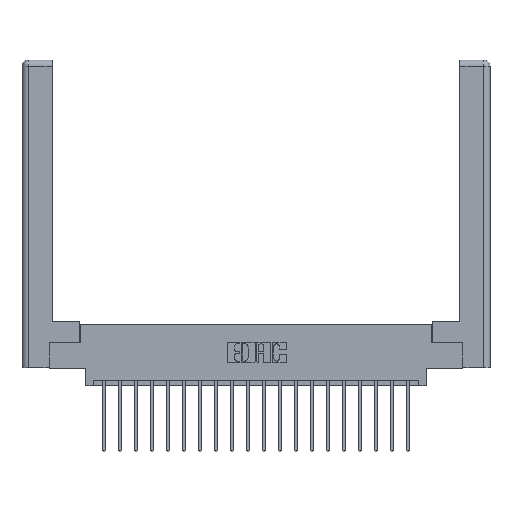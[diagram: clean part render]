
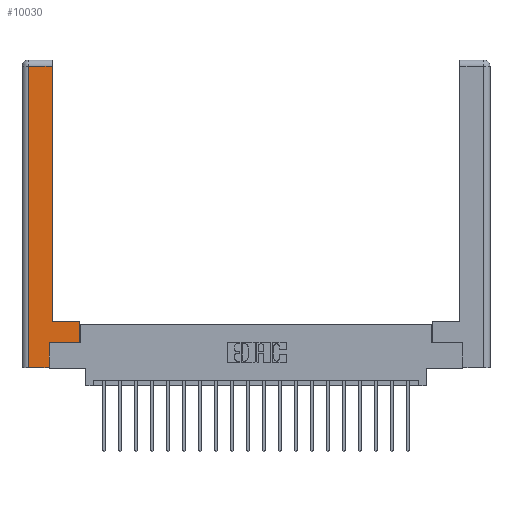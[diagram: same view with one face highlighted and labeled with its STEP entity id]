
A CAD part, top view. The second image highlights one B-rep face of the part: STEP entity #10030.
In plain terms, the highlighted planar face has unit normal (0, 0, 1).
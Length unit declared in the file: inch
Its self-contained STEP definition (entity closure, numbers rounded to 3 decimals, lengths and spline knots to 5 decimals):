
#291 = CARTESIAN_POINT ( 'NONE',  ( 0.265, 0.245, 0. ) ) ;
#354 = VECTOR ( 'NONE', #7674, 39.37008 ) ;
#546 = CARTESIAN_POINT ( 'NONE',  ( 0.0615, 2.94, 0. ) ) ;
#1181 = PLANE ( 'NONE',  #9428 ) ;
#1514 = EDGE_CURVE ( 'NONE', #5510, #20855, #13530, .T. ) ;
#1577 = CARTESIAN_POINT ( 'NONE',  ( 0.295, 2.94, 0. ) ) ;
#1755 = VERTEX_POINT ( 'NONE', #2983 ) ;
#2409 = CARTESIAN_POINT ( 'NONE',  ( 0.265, 0., 0. ) ) ;
#2496 = ORIENTED_EDGE ( 'NONE', *, *, #8917, .T. ) ;
#2958 = VERTEX_POINT ( 'NONE', #291 ) ;
#2983 = CARTESIAN_POINT ( 'NONE',  ( 0.295, 0.45, 0. ) ) ;
#3250 = LINE ( 'NONE', #9101, #7312 ) ;
#3338 = VECTOR ( 'NONE', #19075, 39.37008 ) ;
#3557 = CARTESIAN_POINT ( 'NONE',  ( 0.265, 0., 0. ) ) ;
#3726 = ORIENTED_EDGE ( 'NONE', *, *, #14998, .T. ) ;
#3852 = LINE ( 'NONE', #12488, #3338 ) ;
#4412 = DIRECTION ( 'NONE',  ( 0., 1., 0. ) ) ;
#4414 = DIRECTION ( 'NONE',  ( -1., 0., 0. ) ) ;
#4486 = DIRECTION ( 'NONE',  ( 0., 0., -1. ) ) ;
#4627 = LINE ( 'NONE', #19102, #10732 ) ;
#5510 = VERTEX_POINT ( 'NONE', #15544 ) ;
#5844 = VERTEX_POINT ( 'NONE', #11679 ) ;
#6063 = FACE_OUTER_BOUND ( 'NONE', #18761, .T. ) ;
#6255 = ORIENTED_EDGE ( 'NONE', *, *, #10693, .T. ) ;
#6466 = DIRECTION ( 'NONE',  ( 0., -1., 0. ) ) ;
#6658 = ORIENTED_EDGE ( 'NONE', *, *, #1514, .T. ) ;
#7312 = VECTOR ( 'NONE', #4412, 39.37008 ) ;
#7674 = DIRECTION ( 'NONE',  ( 0., 1., 0. ) ) ;
#8018 = LINE ( 'NONE', #9523, #354 ) ;
#8917 = EDGE_CURVE ( 'NONE', #2958, #19287, #4627, .T. ) ;
#9101 = CARTESIAN_POINT ( 'NONE',  ( 0.565, 0.45, 0. ) ) ;
#9197 = VECTOR ( 'NONE', #13672, 39.37008 ) ;
#9251 = VECTOR ( 'NONE', #16323, 39.37008 ) ;
#9428 = AXIS2_PLACEMENT_3D ( 'NONE', #10957, #4486, #4414 ) ;
#9523 = CARTESIAN_POINT ( 'NONE',  ( 0.295, 3., 0. ) ) ;
#9700 = VECTOR ( 'NONE', #14071, 39.37008 ) ;
#10030 = ADVANCED_FACE ( 'NONE', ( #6063 ), #1181, .F. ) ;
#10693 = EDGE_CURVE ( 'NONE', #19287, #5844, #3250, .T. ) ;
#10732 = VECTOR ( 'NONE', #12814, 39.37008 ) ;
#10761 = ORIENTED_EDGE ( 'NONE', *, *, #15129, .T. ) ;
#10957 = CARTESIAN_POINT ( 'NONE',  ( 0., 0., 0. ) ) ;
#11517 = CARTESIAN_POINT ( 'NONE',  ( 0.565, 0.245, 0. ) ) ;
#11679 = CARTESIAN_POINT ( 'NONE',  ( 0.565, 0.45, 0. ) ) ;
#12003 = EDGE_CURVE ( 'NONE', #1755, #14432, #8018, .T. ) ;
#12488 = CARTESIAN_POINT ( 'NONE',  ( 0.265, 0.245, 0. ) ) ;
#12814 = DIRECTION ( 'NONE',  ( 1., 0., 0. ) ) ;
#13241 = CARTESIAN_POINT ( 'NONE',  ( 0.295, 0.45, 0. ) ) ;
#13530 = LINE ( 'NONE', #2409, #9197 ) ;
#13672 = DIRECTION ( 'NONE',  ( 1., 0., 0. ) ) ;
#13753 = LINE ( 'NONE', #18787, #9700 ) ;
#14071 = DIRECTION ( 'NONE',  ( -1., 0., 0. ) ) ;
#14432 = VERTEX_POINT ( 'NONE', #1577 ) ;
#14606 = LINE ( 'NONE', #13241, #9251 ) ;
#14998 = EDGE_CURVE ( 'NONE', #14432, #15885, #13753, .T. ) ;
#15030 = ORIENTED_EDGE ( 'NONE', *, *, #15098, .T. ) ;
#15098 = EDGE_CURVE ( 'NONE', #20855, #2958, #3852, .T. ) ;
#15129 = EDGE_CURVE ( 'NONE', #15885, #5510, #20163, .T. ) ;
#15544 = CARTESIAN_POINT ( 'NONE',  ( 0.0615, 0., 0. ) ) ;
#15885 = VERTEX_POINT ( 'NONE', #546 ) ;
#16323 = DIRECTION ( 'NONE',  ( -1., 0., 0. ) ) ;
#18761 = EDGE_LOOP ( 'NONE', ( #20225, #3726, #10761, #6658, #15030, #2496, #6255, #20287 ) ) ;
#18787 = CARTESIAN_POINT ( 'NONE',  ( 0.0615, 2.94, 0. ) ) ;
#19075 = DIRECTION ( 'NONE',  ( 0., 1., 0. ) ) ;
#19102 = CARTESIAN_POINT ( 'NONE',  ( 0.565, 0.245, 0. ) ) ;
#19249 = EDGE_CURVE ( 'NONE', #5844, #1755, #14606, .T. ) ;
#19287 = VERTEX_POINT ( 'NONE', #11517 ) ;
#19410 = VECTOR ( 'NONE', #6466, 39.37008 ) ;
#19584 = CARTESIAN_POINT ( 'NONE',  ( 0.0615, 0., 0. ) ) ;
#20163 = LINE ( 'NONE', #19584, #19410 ) ;
#20225 = ORIENTED_EDGE ( 'NONE', *, *, #12003, .T. ) ;
#20287 = ORIENTED_EDGE ( 'NONE', *, *, #19249, .T. ) ;
#20855 = VERTEX_POINT ( 'NONE', #3557 ) ;
